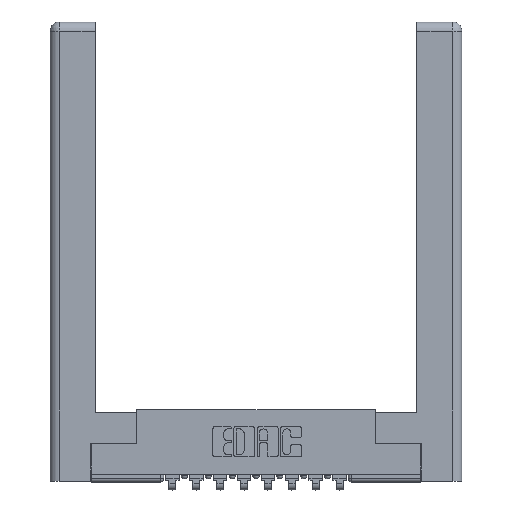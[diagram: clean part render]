
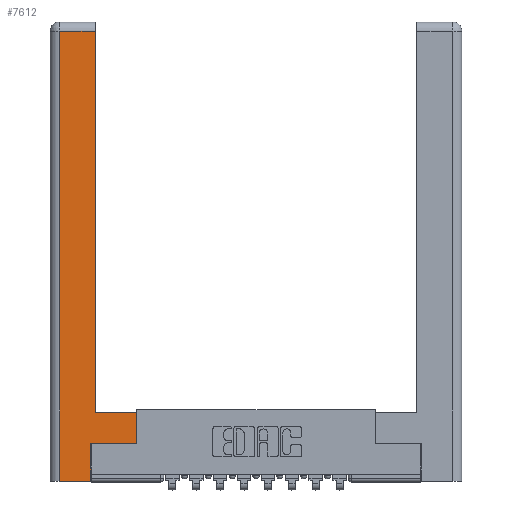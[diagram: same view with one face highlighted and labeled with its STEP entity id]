
A CAD part, top view. The second image highlights one B-rep face of the part: STEP entity #7612.
In plain terms, the highlighted planar face has unit normal (0, 0, 1).
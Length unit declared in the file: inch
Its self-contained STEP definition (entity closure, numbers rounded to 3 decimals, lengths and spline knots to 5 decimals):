
#797 = EDGE_CURVE ( 'NONE', #5879, #9115, #9351, .T. ) ;
#1111 = DIRECTION ( 'NONE',  ( 0., 1., 0. ) ) ;
#1837 = VERTEX_POINT ( 'NONE', #5774 ) ;
#1879 = CARTESIAN_POINT ( 'NONE',  ( 0.265, 0.245, 0. ) ) ;
#1884 = VECTOR ( 'NONE', #8045, 39.37008 ) ;
#2010 = VERTEX_POINT ( 'NONE', #12686 ) ;
#2198 = EDGE_CURVE ( 'NONE', #1837, #5468, #9891, .T. ) ;
#2565 = DIRECTION ( 'NONE',  ( 1., 0., 0. ) ) ;
#2688 = DIRECTION ( 'NONE',  ( -1., 0., 0. ) ) ;
#2823 = CARTESIAN_POINT ( 'NONE',  ( 0.0615, 0., 0. ) ) ;
#3131 = LINE ( 'NONE', #1879, #14292 ) ;
#3148 = ORIENTED_EDGE ( 'NONE', *, *, #7680, .T. ) ;
#3213 = ORIENTED_EDGE ( 'NONE', *, *, #3652, .T. ) ;
#3652 = EDGE_CURVE ( 'NONE', #9115, #9925, #8109, .T. ) ;
#3843 = EDGE_CURVE ( 'NONE', #2010, #9153, #3904, .T. ) ;
#3904 = LINE ( 'NONE', #13189, #4698 ) ;
#4236 = DIRECTION ( 'NONE',  ( -1., 0., 0. ) ) ;
#4698 = VECTOR ( 'NONE', #8546, 39.37008 ) ;
#5312 = VECTOR ( 'NONE', #2688, 39.37008 ) ;
#5316 = EDGE_CURVE ( 'NONE', #5468, #13889, #6725, .T. ) ;
#5411 = LINE ( 'NONE', #9905, #14402 ) ;
#5468 = VERTEX_POINT ( 'NONE', #9997 ) ;
#5485 = PLANE ( 'NONE',  #14174 ) ;
#5702 = ORIENTED_EDGE ( 'NONE', *, *, #797, .T. ) ;
#5774 = CARTESIAN_POINT ( 'NONE',  ( 0.265, 0.245, 0. ) ) ;
#5879 = VERTEX_POINT ( 'NONE', #8744 ) ;
#5905 = CARTESIAN_POINT ( 'NONE',  ( 0.265, 0., 0. ) ) ;
#6725 = LINE ( 'NONE', #11202, #10849 ) ;
#6831 = ORIENTED_EDGE ( 'NONE', *, *, #2198, .T. ) ;
#7035 = CARTESIAN_POINT ( 'NONE',  ( 0.295, 2.94, 0. ) ) ;
#7283 = CARTESIAN_POINT ( 'NONE',  ( 0.565, 0.45, 0. ) ) ;
#7550 = DIRECTION ( 'NONE',  ( 0., 1., 0. ) ) ;
#7612 = ADVANCED_FACE ( 'NONE', ( #7615 ), #5485, .F. ) ;
#7615 = FACE_OUTER_BOUND ( 'NONE', #9273, .T. ) ;
#7617 = ORIENTED_EDGE ( 'NONE', *, *, #5316, .T. ) ;
#7680 = EDGE_CURVE ( 'NONE', #13889, #2010, #5411, .T. ) ;
#8045 = DIRECTION ( 'NONE',  ( 1., 0., 0. ) ) ;
#8092 = CARTESIAN_POINT ( 'NONE',  ( 0.565, 0.245, 0. ) ) ;
#8109 = LINE ( 'NONE', #5905, #1884 ) ;
#8258 = DIRECTION ( 'NONE',  ( 0., -1., 0. ) ) ;
#8326 = ORIENTED_EDGE ( 'NONE', *, *, #8817, .T. ) ;
#8546 = DIRECTION ( 'NONE',  ( 0., 1., 0. ) ) ;
#8744 = CARTESIAN_POINT ( 'NONE',  ( 0.0615, 2.94, 0. ) ) ;
#8817 = EDGE_CURVE ( 'NONE', #9153, #5879, #9399, .T. ) ;
#9115 = VERTEX_POINT ( 'NONE', #2823 ) ;
#9153 = VERTEX_POINT ( 'NONE', #7035 ) ;
#9273 = EDGE_LOOP ( 'NONE', ( #11248, #8326, #5702, #3213, #14355, #6831, #7617, #3148 ) ) ;
#9351 = LINE ( 'NONE', #13856, #11196 ) ;
#9399 = LINE ( 'NONE', #13901, #5312 ) ;
#9758 = DIRECTION ( 'NONE',  ( -1., 0., 0. ) ) ;
#9891 = LINE ( 'NONE', #8092, #11715 ) ;
#9905 = CARTESIAN_POINT ( 'NONE',  ( 0.295, 0.45, 0. ) ) ;
#9925 = VERTEX_POINT ( 'NONE', #10162 ) ;
#9997 = CARTESIAN_POINT ( 'NONE',  ( 0.565, 0.245, 0. ) ) ;
#10162 = CARTESIAN_POINT ( 'NONE',  ( 0.265, 0., 0. ) ) ;
#10849 = VECTOR ( 'NONE', #1111, 39.37008 ) ;
#11196 = VECTOR ( 'NONE', #8258, 39.37008 ) ;
#11202 = CARTESIAN_POINT ( 'NONE',  ( 0.565, 0.45, 0. ) ) ;
#11248 = ORIENTED_EDGE ( 'NONE', *, *, #3843, .T. ) ;
#11715 = VECTOR ( 'NONE', #2565, 39.37008 ) ;
#12686 = CARTESIAN_POINT ( 'NONE',  ( 0.295, 0.45, 0. ) ) ;
#13189 = CARTESIAN_POINT ( 'NONE',  ( 0.295, 3., 0. ) ) ;
#13856 = CARTESIAN_POINT ( 'NONE',  ( 0.0615, 0., 0. ) ) ;
#13889 = VERTEX_POINT ( 'NONE', #7283 ) ;
#13901 = CARTESIAN_POINT ( 'NONE',  ( 0.0615, 2.94, 0. ) ) ;
#14174 = AXIS2_PLACEMENT_3D ( 'NONE', #14525, #14320, #4236 ) ;
#14292 = VECTOR ( 'NONE', #7550, 39.37008 ) ;
#14320 = DIRECTION ( 'NONE',  ( 0., 0., -1. ) ) ;
#14355 = ORIENTED_EDGE ( 'NONE', *, *, #14524, .T. ) ;
#14402 = VECTOR ( 'NONE', #9758, 39.37008 ) ;
#14524 = EDGE_CURVE ( 'NONE', #9925, #1837, #3131, .T. ) ;
#14525 = CARTESIAN_POINT ( 'NONE',  ( 0., 0., 0. ) ) ;
